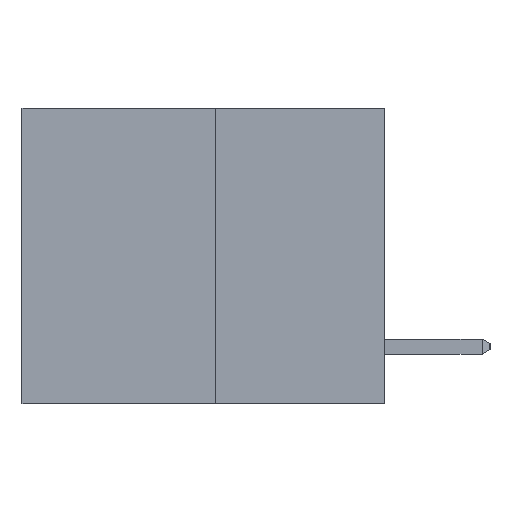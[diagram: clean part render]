
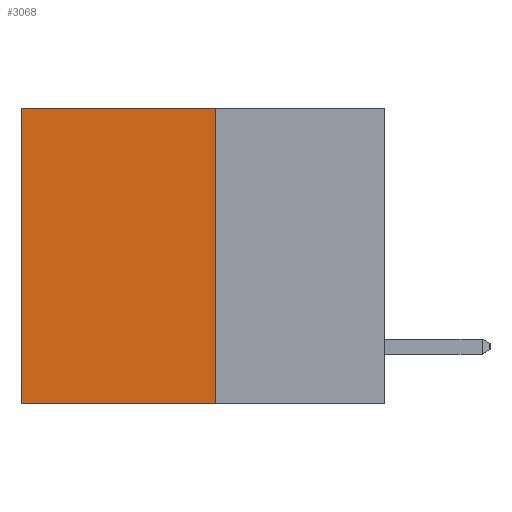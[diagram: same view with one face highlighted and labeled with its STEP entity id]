
A CAD part, left-side view. The second image highlights one B-rep face of the part: STEP entity #3068.
In plain terms, the highlighted planar face has unit normal (-1, 0, 0).
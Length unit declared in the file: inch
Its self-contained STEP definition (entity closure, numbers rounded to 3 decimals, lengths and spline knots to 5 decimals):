
#3 = ORIENTED_EDGE ( 'NONE', *, *, #3921, .T. ) ;
#501 = LINE ( 'NONE', #12151, #4754 ) ;
#927 = CARTESIAN_POINT ( 'NONE',  ( 0.3165, 0.28, -0.49 ) ) ;
#957 = DIRECTION ( 'NONE',  ( 0., 0., -1. ) ) ;
#1020 = VERTEX_POINT ( 'NONE', #7884 ) ;
#1347 = VECTOR ( 'NONE', #13619, 39.37008 ) ;
#3068 = ADVANCED_FACE ( 'NONE', ( #4507 ), #13320, .F. ) ;
#3235 = VERTEX_POINT ( 'NONE', #927 ) ;
#3310 = DIRECTION ( 'NONE',  ( 1., 0., 0. ) ) ;
#3391 = VECTOR ( 'NONE', #9055, 39.37008 ) ;
#3540 = VERTEX_POINT ( 'NONE', #7684 ) ;
#3921 = EDGE_CURVE ( 'NONE', #3540, #10913, #4125, .T. ) ;
#4125 = LINE ( 'NONE', #12905, #11005 ) ;
#4382 = ORIENTED_EDGE ( 'NONE', *, *, #5198, .F. ) ;
#4507 = FACE_OUTER_BOUND ( 'NONE', #5998, .T. ) ;
#4754 = VECTOR ( 'NONE', #5342, 39.37008 ) ;
#5198 = EDGE_CURVE ( 'NONE', #3540, #3235, #501, .T. ) ;
#5342 = DIRECTION ( 'NONE',  ( 0., 0., -1. ) ) ;
#5998 = EDGE_LOOP ( 'NONE', ( #14188, #6763, #4382, #3 ) ) ;
#6374 = LINE ( 'NONE', #6860, #3391 ) ;
#6472 = EDGE_CURVE ( 'NONE', #10913, #1020, #13156, .T. ) ;
#6763 = ORIENTED_EDGE ( 'NONE', *, *, #9551, .F. ) ;
#6860 = CARTESIAN_POINT ( 'NONE',  ( 0.3165, 0.28, -0.49 ) ) ;
#7684 = CARTESIAN_POINT ( 'NONE',  ( 0.3165, 0.28, 0. ) ) ;
#7884 = CARTESIAN_POINT ( 'NONE',  ( 0.3165, 0.6, -0.49 ) ) ;
#9055 = DIRECTION ( 'NONE',  ( 0., 1., 0. ) ) ;
#9551 = EDGE_CURVE ( 'NONE', #3235, #1020, #6374, .T. ) ;
#10039 = CARTESIAN_POINT ( 'NONE',  ( 0.3165, 0.28, -0.49 ) ) ;
#10643 = DIRECTION ( 'NONE',  ( 0., 1., 0. ) ) ;
#10913 = VERTEX_POINT ( 'NONE', #13584 ) ;
#11005 = VECTOR ( 'NONE', #10643, 39.37008 ) ;
#11608 = CARTESIAN_POINT ( 'NONE',  ( 0.3165, 0.6, -0.49 ) ) ;
#12151 = CARTESIAN_POINT ( 'NONE',  ( 0.3165, 0.28, -0.49 ) ) ;
#12544 = AXIS2_PLACEMENT_3D ( 'NONE', #10039, #3310, #957 ) ;
#12905 = CARTESIAN_POINT ( 'NONE',  ( 0.3165, 0.28, 0. ) ) ;
#13156 = LINE ( 'NONE', #11608, #1347 ) ;
#13320 = PLANE ( 'NONE',  #12544 ) ;
#13584 = CARTESIAN_POINT ( 'NONE',  ( 0.3165, 0.6, 0. ) ) ;
#13619 = DIRECTION ( 'NONE',  ( 0., 0., -1. ) ) ;
#14188 = ORIENTED_EDGE ( 'NONE', *, *, #6472, .T. ) ;
